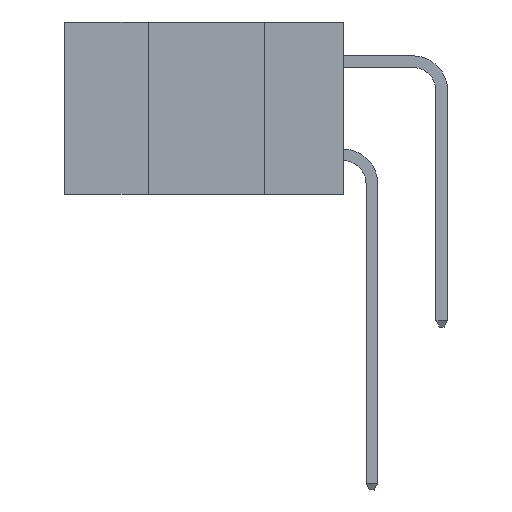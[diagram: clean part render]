
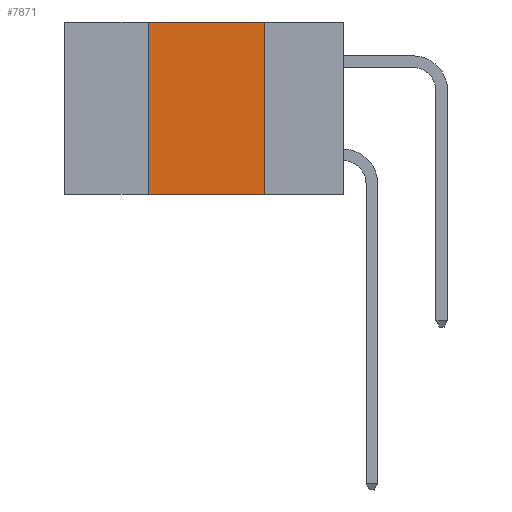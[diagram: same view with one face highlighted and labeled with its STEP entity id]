
A CAD part, left-side view. The second image highlights one B-rep face of the part: STEP entity #7871.
In plain terms, the highlighted planar face has unit normal (-1, 0, 0).
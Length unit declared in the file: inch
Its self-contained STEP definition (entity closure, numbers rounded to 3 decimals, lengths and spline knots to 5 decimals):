
#42 = VECTOR ( 'NONE', #15237, 39.37008 ) ;
#579 = VERTEX_POINT ( 'NONE', #13058 ) ;
#1057 = FACE_OUTER_BOUND ( 'NONE', #11910, .T. ) ;
#1320 = PLANE ( 'NONE',  #13469 ) ;
#1746 = LINE ( 'NONE', #8304, #13211 ) ;
#1876 = EDGE_CURVE ( 'NONE', #10103, #13271, #1746, .T. ) ;
#1948 = VECTOR ( 'NONE', #6982, 39.37008 ) ;
#2416 = VECTOR ( 'NONE', #14220, 39.37008 ) ;
#2536 = CARTESIAN_POINT ( 'NONE',  ( 0., 0.6, 0. ) ) ;
#4469 = DIRECTION ( 'NONE',  ( 0., 0., -1. ) ) ;
#4928 = EDGE_CURVE ( 'NONE', #10005, #13271, #9596, .T. ) ;
#6421 = EDGE_CURVE ( 'NONE', #579, #10103, #15004, .T. ) ;
#6982 = DIRECTION ( 'NONE',  ( 0., -1., 0. ) ) ;
#7871 = ADVANCED_FACE ( 'NONE', ( #1057 ), #1320, .F. ) ;
#8304 = CARTESIAN_POINT ( 'NONE',  ( 0., 0.17, 0. ) ) ;
#8459 = LINE ( 'NONE', #14007, #42 ) ;
#9274 = ORIENTED_EDGE ( 'NONE', *, *, #14647, .F. ) ;
#9347 = ORIENTED_EDGE ( 'NONE', *, *, #1876, .F. ) ;
#9596 = LINE ( 'NONE', #10587, #1948 ) ;
#9938 = ORIENTED_EDGE ( 'NONE', *, *, #4928, .T. ) ;
#10005 = VERTEX_POINT ( 'NONE', #13625 ) ;
#10103 = VERTEX_POINT ( 'NONE', #11389 ) ;
#10587 = CARTESIAN_POINT ( 'NONE',  ( 0., 0.6, -0.37 ) ) ;
#10851 = DIRECTION ( 'NONE',  ( 1., 0., 0. ) ) ;
#11075 = DIRECTION ( 'NONE',  ( 0., 0., -1. ) ) ;
#11365 = CARTESIAN_POINT ( 'NONE',  ( 0., 0.17, -0.37 ) ) ;
#11389 = CARTESIAN_POINT ( 'NONE',  ( 0., 0.17, 0. ) ) ;
#11910 = EDGE_LOOP ( 'NONE', ( #9347, #13266, #9274, #9938 ) ) ;
#13058 = CARTESIAN_POINT ( 'NONE',  ( 0., 0.42, 0. ) ) ;
#13211 = VECTOR ( 'NONE', #4469, 39.37008 ) ;
#13266 = ORIENTED_EDGE ( 'NONE', *, *, #6421, .F. ) ;
#13271 = VERTEX_POINT ( 'NONE', #11365 ) ;
#13469 = AXIS2_PLACEMENT_3D ( 'NONE', #2536, #10851, #11075 ) ;
#13625 = CARTESIAN_POINT ( 'NONE',  ( 0., 0.42, -0.37 ) ) ;
#14007 = CARTESIAN_POINT ( 'NONE',  ( 0., 0.42, 0. ) ) ;
#14220 = DIRECTION ( 'NONE',  ( 0., -1., 0. ) ) ;
#14647 = EDGE_CURVE ( 'NONE', #10005, #579, #8459, .T. ) ;
#15004 = LINE ( 'NONE', #15496, #2416 ) ;
#15237 = DIRECTION ( 'NONE',  ( 0., 0., 1. ) ) ;
#15496 = CARTESIAN_POINT ( 'NONE',  ( 0., 0.6, 0. ) ) ;
